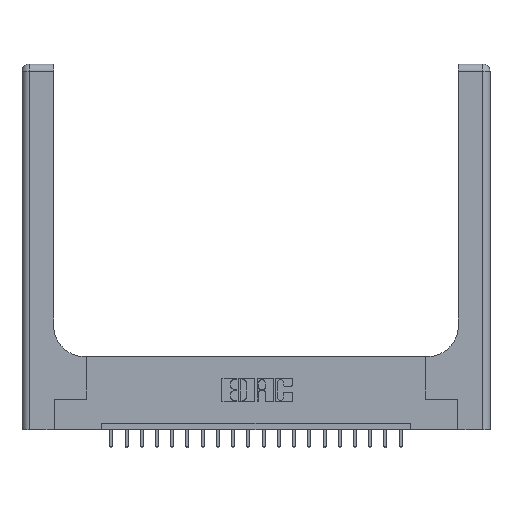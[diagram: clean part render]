
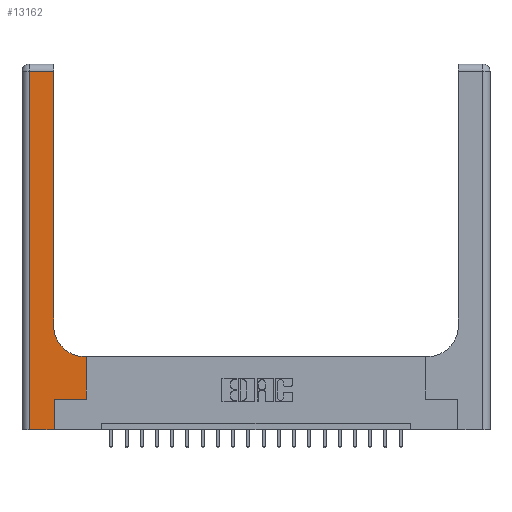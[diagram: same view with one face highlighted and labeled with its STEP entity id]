
A CAD part, top view. The second image highlights one B-rep face of the part: STEP entity #13162.
In plain terms, the highlighted planar face has unit normal (0, 0, 1).
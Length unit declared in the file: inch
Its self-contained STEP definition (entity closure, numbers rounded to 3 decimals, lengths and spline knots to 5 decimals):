
#420 = EDGE_CURVE ( 'NONE', #3782, #2315, #20211, .T. ) ;
#722 = EDGE_LOOP ( 'NONE', ( #6723, #10813, #14065, #15914, #9838, #6278, #16325, #18644, #7517 ) ) ;
#1733 = VERTEX_POINT ( 'NONE', #8500 ) ;
#1815 = LINE ( 'NONE', #13507, #14419 ) ;
#2063 = CARTESIAN_POINT ( 'NONE',  ( 0.528, 0.6, 0.37 ) ) ;
#2209 = VECTOR ( 'NONE', #18562, 39.37008 ) ;
#2315 = VERTEX_POINT ( 'NONE', #11978 ) ;
#3076 = VERTEX_POINT ( 'NONE', #17217 ) ;
#3204 = VECTOR ( 'NONE', #18289, 39.37008 ) ;
#3782 = VERTEX_POINT ( 'NONE', #4852 ) ;
#4181 = VECTOR ( 'NONE', #5960, 39.37008 ) ;
#4784 = DIRECTION ( 'NONE',  ( 0., 1., 0. ) ) ;
#4852 = CARTESIAN_POINT ( 'NONE',  ( 0.51, 0.6, 0.37 ) ) ;
#5859 = CARTESIAN_POINT ( 'NONE',  ( 0., 2.94, 0.37 ) ) ;
#5960 = DIRECTION ( 'NONE',  ( 0., 1., 0. ) ) ;
#5964 = VECTOR ( 'NONE', #4784, 39.37008 ) ;
#6278 = ORIENTED_EDGE ( 'NONE', *, *, #11589, .T. ) ;
#6723 = ORIENTED_EDGE ( 'NONE', *, *, #9614, .T. ) ;
#6934 = CARTESIAN_POINT ( 'NONE',  ( 0., 0., 0.37 ) ) ;
#7249 = VERTEX_POINT ( 'NONE', #13259 ) ;
#7517 = ORIENTED_EDGE ( 'NONE', *, *, #420, .T. ) ;
#7713 = VECTOR ( 'NONE', #18828, 39.37008 ) ;
#8500 = CARTESIAN_POINT ( 'NONE',  ( 0.06, 2.94, 0.37 ) ) ;
#8615 = DIRECTION ( 'NONE',  ( 0., 1., 0. ) ) ;
#8746 = LINE ( 'NONE', #5859, #7713 ) ;
#8776 = DIRECTION ( 'NONE',  ( 1., 0., 0. ) ) ;
#8832 = CARTESIAN_POINT ( 'NONE',  ( 0.528, 0.25, 0.37 ) ) ;
#8885 = LINE ( 'NONE', #12477, #15436 ) ;
#9543 = EDGE_CURVE ( 'NONE', #1733, #3076, #18706, .T. ) ;
#9560 = CARTESIAN_POINT ( 'NONE',  ( 0.26, 3., 0.37 ) ) ;
#9614 = EDGE_CURVE ( 'NONE', #2315, #7249, #11146, .T. ) ;
#9783 = CARTESIAN_POINT ( 'NONE',  ( 0.265, 0., 0.37 ) ) ;
#9838 = ORIENTED_EDGE ( 'NONE', *, *, #12713, .T. ) ;
#10457 = PLANE ( 'NONE',  #17194 ) ;
#10813 = ORIENTED_EDGE ( 'NONE', *, *, #14759, .T. ) ;
#11040 = CARTESIAN_POINT ( 'NONE',  ( 0.265, 0.25, 0.37 ) ) ;
#11069 = VECTOR ( 'NONE', #19787, 39.37008 ) ;
#11146 = LINE ( 'NONE', #9560, #4181 ) ;
#11589 = EDGE_CURVE ( 'NONE', #15172, #20584, #15268, .T. ) ;
#11806 = CARTESIAN_POINT ( 'NONE',  ( 0.06, 3., 0.37 ) ) ;
#11974 = VERTEX_POINT ( 'NONE', #13217 ) ;
#11978 = CARTESIAN_POINT ( 'NONE',  ( 0.26, 0.85, 0.37 ) ) ;
#12062 = CARTESIAN_POINT ( 'NONE',  ( 0.51, 0.85, 0.37 ) ) ;
#12087 = VERTEX_POINT ( 'NONE', #2063 ) ;
#12477 = CARTESIAN_POINT ( 'NONE',  ( 0.26, 0.6, 0.37 ) ) ;
#12713 = EDGE_CURVE ( 'NONE', #11974, #15172, #19337, .T. ) ;
#13162 = ADVANCED_FACE ( 'NONE', ( #18848 ), #10457, .F. ) ;
#13217 = CARTESIAN_POINT ( 'NONE',  ( 0.265, 0., 0.37 ) ) ;
#13259 = CARTESIAN_POINT ( 'NONE',  ( 0.26, 2.94, 0.37 ) ) ;
#13378 = EDGE_CURVE ( 'NONE', #3076, #11974, #14576, .T. ) ;
#13507 = CARTESIAN_POINT ( 'NONE',  ( 0.528, 0.25, 0.37 ) ) ;
#13771 = CARTESIAN_POINT ( 'NONE',  ( 0.265, 0.25, 0.37 ) ) ;
#14065 = ORIENTED_EDGE ( 'NONE', *, *, #9543, .T. ) ;
#14419 = VECTOR ( 'NONE', #8615, 39.37008 ) ;
#14576 = LINE ( 'NONE', #6934, #11069 ) ;
#14759 = EDGE_CURVE ( 'NONE', #7249, #1733, #8746, .T. ) ;
#15040 = DIRECTION ( 'NONE',  ( 0., 0., -1. ) ) ;
#15172 = VERTEX_POINT ( 'NONE', #11040 ) ;
#15268 = LINE ( 'NONE', #13771, #2209 ) ;
#15436 = VECTOR ( 'NONE', #18965, 39.37008 ) ;
#15449 = AXIS2_PLACEMENT_3D ( 'NONE', #12062, #15040, #8776 ) ;
#15914 = ORIENTED_EDGE ( 'NONE', *, *, #13378, .T. ) ;
#16325 = ORIENTED_EDGE ( 'NONE', *, *, #20058, .T. ) ;
#17036 = DIRECTION ( 'NONE',  ( -1., 0., 0. ) ) ;
#17194 = AXIS2_PLACEMENT_3D ( 'NONE', #20134, #20246, #17036 ) ;
#17217 = CARTESIAN_POINT ( 'NONE',  ( 0.06, 0., 0.37 ) ) ;
#18289 = DIRECTION ( 'NONE',  ( 0., -1., 0. ) ) ;
#18562 = DIRECTION ( 'NONE',  ( 1., 0., 0. ) ) ;
#18644 = ORIENTED_EDGE ( 'NONE', *, *, #21012, .T. ) ;
#18706 = LINE ( 'NONE', #11806, #3204 ) ;
#18828 = DIRECTION ( 'NONE',  ( -1., 0., 0. ) ) ;
#18848 = FACE_OUTER_BOUND ( 'NONE', #722, .T. ) ;
#18965 = DIRECTION ( 'NONE',  ( -1., 0., 0. ) ) ;
#19337 = LINE ( 'NONE', #9783, #5964 ) ;
#19787 = DIRECTION ( 'NONE',  ( 1., 0., 0. ) ) ;
#20058 = EDGE_CURVE ( 'NONE', #20584, #12087, #1815, .T. ) ;
#20134 = CARTESIAN_POINT ( 'NONE',  ( 0., 3., 0.37 ) ) ;
#20211 = CIRCLE ( 'NONE', #15449, 0.25 ) ;
#20246 = DIRECTION ( 'NONE',  ( 0., 0., -1. ) ) ;
#20584 = VERTEX_POINT ( 'NONE', #8832 ) ;
#21012 = EDGE_CURVE ( 'NONE', #12087, #3782, #8885, .T. ) ;
